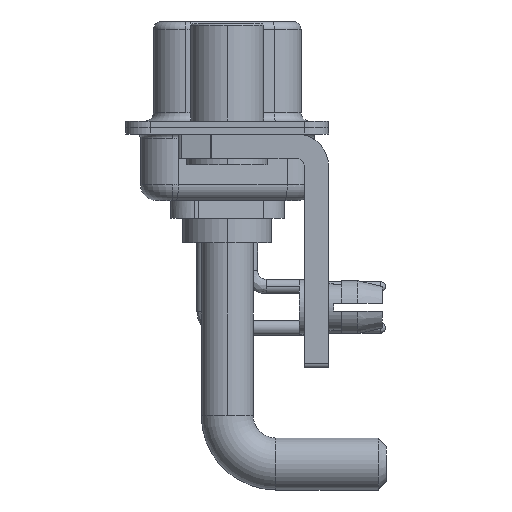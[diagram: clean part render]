
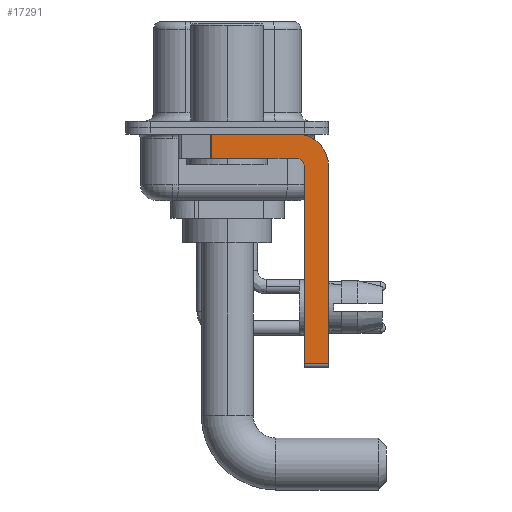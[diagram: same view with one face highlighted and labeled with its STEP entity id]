
A CAD part, left-side view. The second image highlights one B-rep face of the part: STEP entity #17291.
In plain terms, the highlighted planar face has unit normal (-1, 0, 0).
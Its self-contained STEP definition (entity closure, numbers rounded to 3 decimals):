
#259 = LINE ( 'NONE', #24462, #8910 ) ;
#277 = VECTOR ( 'NONE', #8966, 1000. ) ;
#913 = ORIENTED_EDGE ( 'NONE', *, *, #22386, .F. ) ;
#1370 = CARTESIAN_POINT ( 'NONE',  ( -2.9, -6.25, -14.55 ) ) ;
#1512 = DIRECTION ( 'NONE',  ( 0., -1., 0. ) ) ;
#1666 = CARTESIAN_POINT ( 'NONE',  ( -2.9, 3., -0.4 ) ) ;
#1723 = LINE ( 'NONE', #6803, #12346 ) ;
#1844 = VERTEX_POINT ( 'NONE', #25990 ) ;
#2115 = EDGE_CURVE ( 'NONE', #26701, #12979, #8526, .T. ) ;
#2257 = CARTESIAN_POINT ( 'NONE',  ( -2.9, -4.25, -2.4 ) ) ;
#2520 = CARTESIAN_POINT ( 'NONE',  ( -2.9, -4.75, -2.4 ) ) ;
#2662 = DIRECTION ( 'NONE',  ( 0., 0., 1. ) ) ;
#4058 = LINE ( 'NONE', #1666, #5741 ) ;
#4275 = AXIS2_PLACEMENT_3D ( 'NONE', #2257, #24076, #21695 ) ;
#4376 = CARTESIAN_POINT ( 'NONE',  ( -2.9, 0.978, -1.9 ) ) ;
#5529 = CARTESIAN_POINT ( 'NONE',  ( -2.9, -6.25, -2.4 ) ) ;
#5741 = VECTOR ( 'NONE', #1512, 1000. ) ;
#5766 = LINE ( 'NONE', #29963, #20653 ) ;
#6421 = ORIENTED_EDGE ( 'NONE', *, *, #20441, .F. ) ;
#6585 = EDGE_CURVE ( 'NONE', #1844, #25602, #1723, .T. ) ;
#6803 = CARTESIAN_POINT ( 'NONE',  ( -2.9, -4.25, -1.9 ) ) ;
#7251 = DIRECTION ( 'NONE',  ( 0., 0., -1. ) ) ;
#7283 = CARTESIAN_POINT ( 'NONE',  ( -2.9, -4.75, -14.8 ) ) ;
#7794 = EDGE_CURVE ( 'NONE', #12979, #28138, #11519, .T. ) ;
#8526 = CIRCLE ( 'NONE', #15640, 2. ) ;
#8910 = VECTOR ( 'NONE', #7251, 1000. ) ;
#8966 = DIRECTION ( 'NONE',  ( 0., 0., -1. ) ) ;
#8967 = ORIENTED_EDGE ( 'NONE', *, *, #2115, .F. ) ;
#10075 = PLANE ( 'NONE',  #29568 ) ;
#10690 = VERTEX_POINT ( 'NONE', #11544 ) ;
#10908 = DIRECTION ( 'NONE',  ( 1., 0., 0. ) ) ;
#11519 = LINE ( 'NONE', #21071, #277 ) ;
#11544 = CARTESIAN_POINT ( 'NONE',  ( -2.9, 0.978, -0.4 ) ) ;
#11730 = VERTEX_POINT ( 'NONE', #15978 ) ;
#11762 = ORIENTED_EDGE ( 'NONE', *, *, #24674, .T. ) ;
#12346 = VECTOR ( 'NONE', #28776, 1000. ) ;
#12434 = ORIENTED_EDGE ( 'NONE', *, *, #18158, .F. ) ;
#12778 = DIRECTION ( 'NONE',  ( 0., 0., -1. ) ) ;
#12979 = VERTEX_POINT ( 'NONE', #5529 ) ;
#15640 = AXIS2_PLACEMENT_3D ( 'NONE', #25399, #10908, #16312 ) ;
#15978 = CARTESIAN_POINT ( 'NONE',  ( -2.9, -4.75, -14.55 ) ) ;
#16312 = DIRECTION ( 'NONE',  ( 0., 0., -1. ) ) ;
#16889 = VECTOR ( 'NONE', #2662, 1000. ) ;
#17291 = ADVANCED_FACE ( 'NONE', ( #29498 ), #10075, .F. ) ;
#17712 = CARTESIAN_POINT ( 'NONE',  ( -2.9, -4.25, -2.4 ) ) ;
#18158 = EDGE_CURVE ( 'NONE', #11730, #24949, #26716, .T. ) ;
#19788 = DIRECTION ( 'NONE',  ( 1., 0., 0. ) ) ;
#20441 = EDGE_CURVE ( 'NONE', #10690, #26701, #4058, .T. ) ;
#20653 = VECTOR ( 'NONE', #25200, 1000. ) ;
#21071 = CARTESIAN_POINT ( 'NONE',  ( -2.9, -6.25, -2.4 ) ) ;
#21695 = DIRECTION ( 'NONE',  ( 0., 0., 1. ) ) ;
#22386 = EDGE_CURVE ( 'NONE', #24949, #1844, #26141, .T. ) ;
#24056 = EDGE_CURVE ( 'NONE', #10690, #25602, #259, .T. ) ;
#24076 = DIRECTION ( 'NONE',  ( -1., 0., 0. ) ) ;
#24462 = CARTESIAN_POINT ( 'NONE',  ( -2.9, 0.978, -1.9 ) ) ;
#24674 = EDGE_CURVE ( 'NONE', #11730, #28138, #5766, .T. ) ;
#24949 = VERTEX_POINT ( 'NONE', #2520 ) ;
#25200 = DIRECTION ( 'NONE',  ( 0., -1., 0. ) ) ;
#25399 = CARTESIAN_POINT ( 'NONE',  ( -2.9, -4.25, -2.4 ) ) ;
#25602 = VERTEX_POINT ( 'NONE', #4376 ) ;
#25687 = ORIENTED_EDGE ( 'NONE', *, *, #6585, .F. ) ;
#25990 = CARTESIAN_POINT ( 'NONE',  ( -2.9, -4.25, -1.9 ) ) ;
#26005 = ORIENTED_EDGE ( 'NONE', *, *, #7794, .F. ) ;
#26141 = CIRCLE ( 'NONE', #4275, 0.5 ) ;
#26572 = CARTESIAN_POINT ( 'NONE',  ( -2.9, -4.25, -0.4 ) ) ;
#26701 = VERTEX_POINT ( 'NONE', #26572 ) ;
#26716 = LINE ( 'NONE', #7283, #16889 ) ;
#28138 = VERTEX_POINT ( 'NONE', #1370 ) ;
#28501 = EDGE_LOOP ( 'NONE', ( #6421, #30762, #25687, #913, #12434, #11762, #26005, #8967 ) ) ;
#28776 = DIRECTION ( 'NONE',  ( 0., 1., 0. ) ) ;
#29498 = FACE_OUTER_BOUND ( 'NONE', #28501, .T. ) ;
#29568 = AXIS2_PLACEMENT_3D ( 'NONE', #17712, #19788, #12778 ) ;
#29963 = CARTESIAN_POINT ( 'NONE',  ( -2.9, -4.25, -14.55 ) ) ;
#30762 = ORIENTED_EDGE ( 'NONE', *, *, #24056, .T. ) ;
